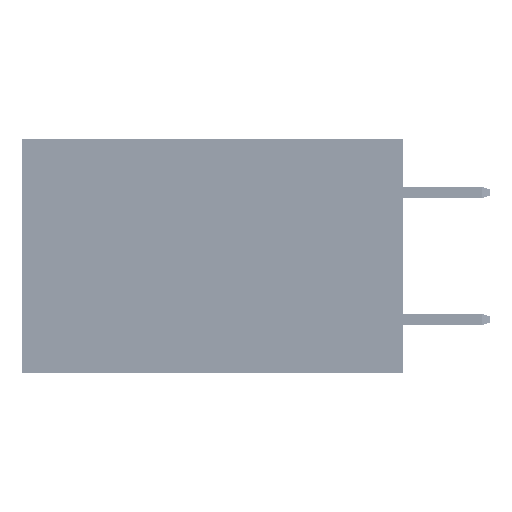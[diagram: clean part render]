
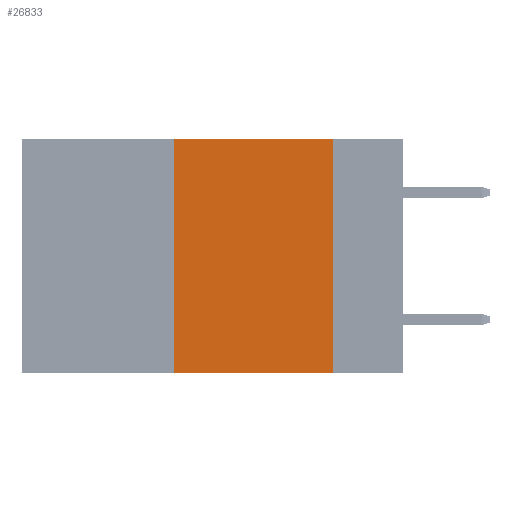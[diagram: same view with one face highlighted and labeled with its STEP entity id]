
A CAD part, left-side view. The second image highlights one B-rep face of the part: STEP entity #26833.
In plain terms, the highlighted planar face has unit normal (-1, 0, 0).
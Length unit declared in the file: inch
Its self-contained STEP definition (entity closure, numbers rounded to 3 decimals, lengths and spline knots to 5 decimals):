
#268 = CARTESIAN_POINT ( 'NONE',  ( 0., 0.6, -0.37 ) ) ;
#1491 = CARTESIAN_POINT ( 'NONE',  ( 0., 0.6, 0. ) ) ;
#3145 = EDGE_CURVE ( 'NONE', #17199, #28965, #39024, .T. ) ;
#8174 = VECTOR ( 'NONE', #16321, 39.37008 ) ;
#8744 = VECTOR ( 'NONE', #45717, 39.37008 ) ;
#9410 = PLANE ( 'NONE',  #36237 ) ;
#10142 = CARTESIAN_POINT ( 'NONE',  ( 0., 0.36, 0. ) ) ;
#12656 = LINE ( 'NONE', #40752, #8174 ) ;
#13706 = CARTESIAN_POINT ( 'NONE',  ( 0., 0.11, -0.37 ) ) ;
#15210 = VERTEX_POINT ( 'NONE', #28141 ) ;
#16321 = DIRECTION ( 'NONE',  ( 0., 0., -1. ) ) ;
#17199 = VERTEX_POINT ( 'NONE', #30657 ) ;
#17724 = DIRECTION ( 'NONE',  ( 0., 0., -1. ) ) ;
#22746 = ORIENTED_EDGE ( 'NONE', *, *, #31160, .F. ) ;
#25192 = EDGE_CURVE ( 'NONE', #36953, #15210, #37127, .T. ) ;
#25260 = CARTESIAN_POINT ( 'NONE',  ( 0., 0.6, 0. ) ) ;
#26254 = LINE ( 'NONE', #10142, #31958 ) ;
#26833 = ADVANCED_FACE ( 'NONE', ( #45052 ), #9410, .F. ) ;
#28141 = CARTESIAN_POINT ( 'NONE',  ( 0., 0.11, 0. ) ) ;
#28965 = VERTEX_POINT ( 'NONE', #13706 ) ;
#30657 = CARTESIAN_POINT ( 'NONE',  ( 0., 0.36, -0.37 ) ) ;
#31160 = EDGE_CURVE ( 'NONE', #15210, #28965, #12656, .T. ) ;
#31756 = EDGE_LOOP ( 'NONE', ( #22746, #49904, #47290, #39903 ) ) ;
#31958 = VECTOR ( 'NONE', #34324, 39.37008 ) ;
#34324 = DIRECTION ( 'NONE',  ( 0., 0., 1. ) ) ;
#36237 = AXIS2_PLACEMENT_3D ( 'NONE', #25260, #37233, #17724 ) ;
#36953 = VERTEX_POINT ( 'NONE', #43493 ) ;
#37127 = LINE ( 'NONE', #1491, #8744 ) ;
#37233 = DIRECTION ( 'NONE',  ( 1., 0., 0. ) ) ;
#39024 = LINE ( 'NONE', #268, #44545 ) ;
#39816 = EDGE_CURVE ( 'NONE', #17199, #36953, #26254, .T. ) ;
#39903 = ORIENTED_EDGE ( 'NONE', *, *, #3145, .T. ) ;
#40752 = CARTESIAN_POINT ( 'NONE',  ( 0., 0.11, 0. ) ) ;
#43493 = CARTESIAN_POINT ( 'NONE',  ( 0., 0.36, 0. ) ) ;
#44545 = VECTOR ( 'NONE', #48647, 39.37008 ) ;
#45052 = FACE_OUTER_BOUND ( 'NONE', #31756, .T. ) ;
#45717 = DIRECTION ( 'NONE',  ( 0., -1., 0. ) ) ;
#47290 = ORIENTED_EDGE ( 'NONE', *, *, #39816, .F. ) ;
#48647 = DIRECTION ( 'NONE',  ( 0., -1., 0. ) ) ;
#49904 = ORIENTED_EDGE ( 'NONE', *, *, #25192, .F. ) ;
